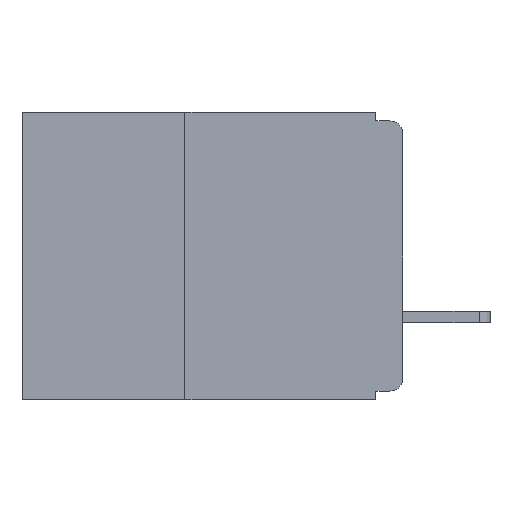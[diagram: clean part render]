
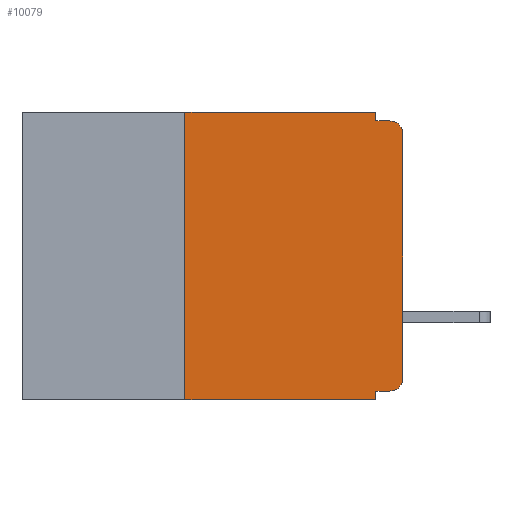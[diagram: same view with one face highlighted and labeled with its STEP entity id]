
A CAD part, left-side view. The second image highlights one B-rep face of the part: STEP entity #10079.
In plain terms, the highlighted planar face has unit normal (-1, 0, 0).
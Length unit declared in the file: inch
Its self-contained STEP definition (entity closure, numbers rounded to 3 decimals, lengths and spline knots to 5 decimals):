
#116 = ORIENTED_EDGE ( 'NONE', *, *, #9384, .T. ) ;
#216 = DIRECTION ( 'NONE',  ( 0., -1., 0. ) ) ;
#293 = CARTESIAN_POINT ( 'NONE',  ( 0., 0.015, -0.32 ) ) ;
#444 = EDGE_CURVE ( 'NONE', #1495, #12329, #8024, .T. ) ;
#463 = ORIENTED_EDGE ( 'NONE', *, *, #7579, .F. ) ;
#584 = VERTEX_POINT ( 'NONE', #8507 ) ;
#675 = CARTESIAN_POINT ( 'NONE',  ( 0., 0.031, 0. ) ) ;
#678 = ORIENTED_EDGE ( 'NONE', *, *, #10634, .T. ) ;
#827 = ORIENTED_EDGE ( 'NONE', *, *, #12776, .F. ) ;
#875 = ORIENTED_EDGE ( 'NONE', *, *, #444, .T. ) ;
#920 = AXIS2_PLACEMENT_3D ( 'NONE', #2412, #10306, #3603 ) ;
#933 = CARTESIAN_POINT ( 'NONE',  ( 0., 0., -0.305 ) ) ;
#1382 = CARTESIAN_POINT ( 'NONE',  ( 0., 0.015, -0.305 ) ) ;
#1430 = CARTESIAN_POINT ( 'NONE',  ( 0., 0.25, -0.33 ) ) ;
#1495 = VERTEX_POINT ( 'NONE', #11241 ) ;
#1578 = DIRECTION ( 'NONE',  ( 0., 0., -1. ) ) ;
#1708 = VECTOR ( 'NONE', #9495, 39.37008 ) ;
#2228 = CARTESIAN_POINT ( 'NONE',  ( 0., 0., 0. ) ) ;
#2369 = VERTEX_POINT ( 'NONE', #13951 ) ;
#2412 = CARTESIAN_POINT ( 'NONE',  ( 0., 0.015, -0.025 ) ) ;
#2650 = DIRECTION ( 'NONE',  ( 0., 0., -1. ) ) ;
#2653 = CARTESIAN_POINT ( 'NONE',  ( 0., 0.031, -0.01 ) ) ;
#2902 = DIRECTION ( 'NONE',  ( 0., 0., -1. ) ) ;
#2905 = CIRCLE ( 'NONE', #10082, 0.015 ) ;
#2969 = VERTEX_POINT ( 'NONE', #675 ) ;
#3028 = VECTOR ( 'NONE', #9635, 39.37008 ) ;
#3145 = VERTEX_POINT ( 'NONE', #2653 ) ;
#3537 = VECTOR ( 'NONE', #5789, 39.37008 ) ;
#3603 = DIRECTION ( 'NONE',  ( 0., 0., -1. ) ) ;
#3961 = CARTESIAN_POINT ( 'NONE',  ( 0., 0.437, 0. ) ) ;
#4234 = VECTOR ( 'NONE', #10318, 39.37008 ) ;
#4251 = CARTESIAN_POINT ( 'NONE',  ( 0., 0.031, -0.33 ) ) ;
#4990 = CARTESIAN_POINT ( 'NONE',  ( 0., 0.031, -0.32 ) ) ;
#5674 = VECTOR ( 'NONE', #216, 39.37008 ) ;
#5789 = DIRECTION ( 'NONE',  ( 0., 0., 1. ) ) ;
#5873 = EDGE_LOOP ( 'NONE', ( #7165, #116, #463, #10957, #13066, #11393, #875, #827, #9031, #678 ) ) ;
#5936 = CARTESIAN_POINT ( 'NONE',  ( 0., 0., -0.32 ) ) ;
#6144 = LINE ( 'NONE', #8626, #13694 ) ;
#6280 = PLANE ( 'NONE',  #11255 ) ;
#6603 = LINE ( 'NONE', #2228, #3537 ) ;
#6618 = EDGE_CURVE ( 'NONE', #11037, #584, #6603, .T. ) ;
#6936 = VECTOR ( 'NONE', #13689, 39.37008 ) ;
#7059 = FACE_OUTER_BOUND ( 'NONE', #5873, .T. ) ;
#7162 = CARTESIAN_POINT ( 'NONE',  ( 0., 0.015, -0.01 ) ) ;
#7165 = ORIENTED_EDGE ( 'NONE', *, *, #6618, .T. ) ;
#7339 = VERTEX_POINT ( 'NONE', #7162 ) ;
#7490 = CARTESIAN_POINT ( 'NONE',  ( 0., 0.437, -0.33 ) ) ;
#7579 = EDGE_CURVE ( 'NONE', #3145, #7339, #12493, .T. ) ;
#8024 = LINE ( 'NONE', #7490, #10181 ) ;
#8102 = VERTEX_POINT ( 'NONE', #4990 ) ;
#8507 = CARTESIAN_POINT ( 'NONE',  ( 0., 0., -0.025 ) ) ;
#8553 = DIRECTION ( 'NONE',  ( 1., 0., 0. ) ) ;
#8626 = CARTESIAN_POINT ( 'NONE',  ( 0., 0.031, 0. ) ) ;
#8628 = EDGE_CURVE ( 'NONE', #12745, #8102, #12764, .T. ) ;
#8667 = LINE ( 'NONE', #10538, #5674 ) ;
#8797 = CARTESIAN_POINT ( 'NONE',  ( 0., 0., -0.01 ) ) ;
#9031 = ORIENTED_EDGE ( 'NONE', *, *, #8628, .F. ) ;
#9384 = EDGE_CURVE ( 'NONE', #584, #7339, #13473, .T. ) ;
#9452 = DIRECTION ( 'NONE',  ( -1., 0., 0. ) ) ;
#9495 = DIRECTION ( 'NONE',  ( 0., 0., 1. ) ) ;
#9504 = EDGE_CURVE ( 'NONE', #2369, #2969, #8667, .T. ) ;
#9589 = CARTESIAN_POINT ( 'NONE',  ( 0., 0.031, -0.33 ) ) ;
#9635 = DIRECTION ( 'NONE',  ( 0., 0., -1. ) ) ;
#10079 = ADVANCED_FACE ( 'NONE', ( #7059 ), #6280, .F. ) ;
#10082 = AXIS2_PLACEMENT_3D ( 'NONE', #1382, #9452, #2650 ) ;
#10181 = VECTOR ( 'NONE', #14087, 39.37008 ) ;
#10306 = DIRECTION ( 'NONE',  ( -1., 0., 0. ) ) ;
#10318 = DIRECTION ( 'NONE',  ( 0., 1., 0. ) ) ;
#10538 = CARTESIAN_POINT ( 'NONE',  ( 0., 0.437, 0. ) ) ;
#10634 = EDGE_CURVE ( 'NONE', #12745, #11037, #2905, .T. ) ;
#10957 = ORIENTED_EDGE ( 'NONE', *, *, #12827, .F. ) ;
#11037 = VERTEX_POINT ( 'NONE', #933 ) ;
#11241 = CARTESIAN_POINT ( 'NONE',  ( 0., 0.25, -0.33 ) ) ;
#11255 = AXIS2_PLACEMENT_3D ( 'NONE', #3961, #8553, #1578 ) ;
#11393 = ORIENTED_EDGE ( 'NONE', *, *, #12664, .F. ) ;
#11835 = LINE ( 'NONE', #9589, #3028 ) ;
#12329 = VERTEX_POINT ( 'NONE', #4251 ) ;
#12493 = LINE ( 'NONE', #8797, #6936 ) ;
#12664 = EDGE_CURVE ( 'NONE', #1495, #2369, #12704, .T. ) ;
#12704 = LINE ( 'NONE', #1430, #1708 ) ;
#12745 = VERTEX_POINT ( 'NONE', #293 ) ;
#12764 = LINE ( 'NONE', #5936, #4234 ) ;
#12776 = EDGE_CURVE ( 'NONE', #8102, #12329, #11835, .T. ) ;
#12827 = EDGE_CURVE ( 'NONE', #2969, #3145, #6144, .T. ) ;
#13066 = ORIENTED_EDGE ( 'NONE', *, *, #9504, .F. ) ;
#13473 = CIRCLE ( 'NONE', #920, 0.015 ) ;
#13689 = DIRECTION ( 'NONE',  ( 0., -1., 0. ) ) ;
#13694 = VECTOR ( 'NONE', #2902, 39.37008 ) ;
#13951 = CARTESIAN_POINT ( 'NONE',  ( 0., 0.25, 0. ) ) ;
#14087 = DIRECTION ( 'NONE',  ( 0., -1., 0. ) ) ;
